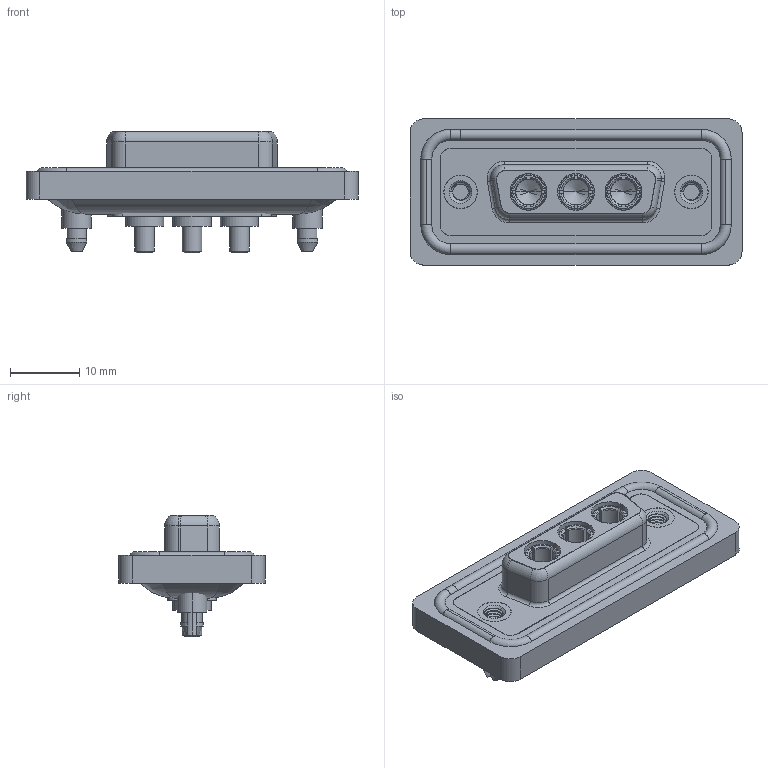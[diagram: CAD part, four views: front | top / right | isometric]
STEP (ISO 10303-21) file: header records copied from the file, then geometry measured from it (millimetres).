
FILE_DESCRIPTION (( 'STEP AP203' ), '1' );
FILE_NAME ('628W3W3-624-2ND.STEP', '2024-03-22T15:05:55', ( '' ), ( '' ), 'SwSTEP 2.0', 'SolidWorks 2023', '' );
FILE_SCHEMA (( 'CONFIG_CONTROL_DESIGN' ));
Length unit declared in the file: millimetre
Products named in the file (7): Power Socket_20A S; 628Combo Housing_3W3; 628Combo Shell Front_15 Contacts; 628W3W3-624-2ND; 628Combo Shell Rear_15 Contacts; 628Combo Threaded Boardlock_D; 628Combo Waterproof Housing_15 Contacts
Assembly tree (9 placements, depth 2):
  628W3W3-624-2ND
    628Combo Housing_3W3
    628Combo Waterproof Housing_15 Contacts
    628Combo Shell Front_15 Contacts
    628Combo Shell Rear_15 Contacts
    628Combo Threaded Boardlock_D  x2
    Power Socket_20A S  x3
Bounding box: 47.9 x 21.1 x 17.55 mm (x, y, z)
Volume: 6161.6 mm3; surface area: 10077.8 mm2
Topology: 13 solids, 13 shells, 674 faces, 1717 edges, 1089 vertices
Faces by surface type: cylinder 305, plane 208, torus 83, cone 63, bspline 15
Entity records: 17508 total; most frequent: CARTESIAN_POINT 5417, DIRECTION 2453, ORIENTED_EDGE 2344, EDGE_CURVE 1172, AXIS2_PLACEMENT_3D 974, VERTEX_POINT 744, EDGE_LOOP 516, VECTOR 505
